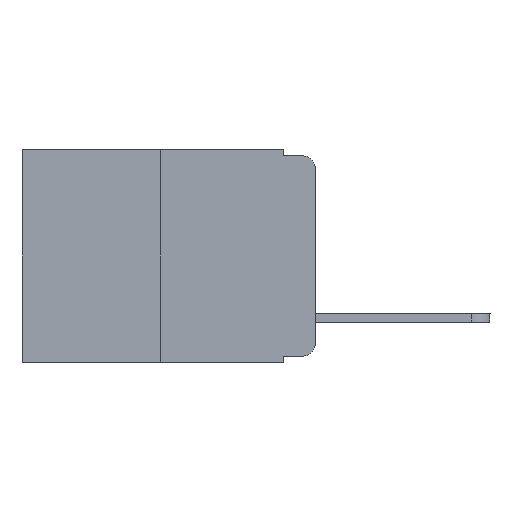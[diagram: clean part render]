
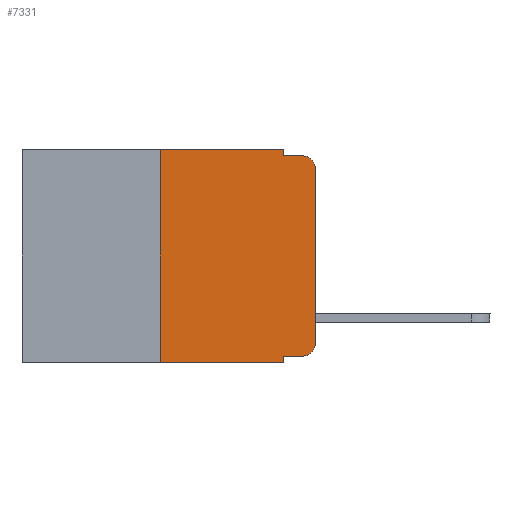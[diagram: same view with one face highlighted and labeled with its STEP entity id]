
A CAD part, left-side view. The second image highlights one B-rep face of the part: STEP entity #7331.
In plain terms, the highlighted planar face has unit normal (-1, 0, 0).
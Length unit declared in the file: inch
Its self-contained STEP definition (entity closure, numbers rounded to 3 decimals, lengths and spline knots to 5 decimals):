
#117 = CARTESIAN_POINT ( 'NONE',  ( 0., 0.473, 0. ) ) ;
#361 = VERTEX_POINT ( 'NONE', #13774 ) ;
#430 = DIRECTION ( 'NONE',  ( 1., 0., 0. ) ) ;
#773 = ORIENTED_EDGE ( 'NONE', *, *, #13720, .T. ) ;
#1698 = ORIENTED_EDGE ( 'NONE', *, *, #6007, .F. ) ;
#1771 = CARTESIAN_POINT ( 'NONE',  ( 0., 0.051, 0. ) ) ;
#1919 = CARTESIAN_POINT ( 'NONE',  ( 0., 0.051, -0.343 ) ) ;
#2036 = EDGE_CURVE ( 'NONE', #12910, #7004, #12169, .T. ) ;
#2043 = AXIS2_PLACEMENT_3D ( 'NONE', #8838, #430, #16953 ) ;
#2101 = VECTOR ( 'NONE', #10260, 39.37008 ) ;
#2117 = FACE_OUTER_BOUND ( 'NONE', #2971, .T. ) ;
#2604 = LINE ( 'NONE', #15202, #16610 ) ;
#2971 = EDGE_LOOP ( 'NONE', ( #773, #12628, #6554, #6378, #11436, #1698, #15024, #17090, #4696, #16770 ) ) ;
#3164 = EDGE_CURVE ( 'NONE', #16800, #361, #15571, .T. ) ;
#3185 = VERTEX_POINT ( 'NONE', #11881 ) ;
#3512 = CARTESIAN_POINT ( 'NONE',  ( 0., 0.02, -0.03 ) ) ;
#3571 = AXIS2_PLACEMENT_3D ( 'NONE', #11490, #14267, #6205 ) ;
#3693 = DIRECTION ( 'NONE',  ( -1., 0., 0. ) ) ;
#3844 = CARTESIAN_POINT ( 'NONE',  ( 0., 0.051, 0. ) ) ;
#3941 = VERTEX_POINT ( 'NONE', #5754 ) ;
#3953 = DIRECTION ( 'NONE',  ( 0., -1., 0. ) ) ;
#3967 = CARTESIAN_POINT ( 'NONE',  ( 0., 0.051, 0. ) ) ;
#4130 = VECTOR ( 'NONE', #16663, 39.37008 ) ;
#4312 = DIRECTION ( 'NONE',  ( 0., -1., 0. ) ) ;
#4548 = PLANE ( 'NONE',  #2043 ) ;
#4601 = DIRECTION ( 'NONE',  ( 0., 0., -1. ) ) ;
#4696 = ORIENTED_EDGE ( 'NONE', *, *, #11594, .T. ) ;
#4795 = VECTOR ( 'NONE', #3953, 39.37008 ) ;
#4859 = CARTESIAN_POINT ( 'NONE',  ( 0., 0., 0. ) ) ;
#4917 = LINE ( 'NONE', #117, #8762 ) ;
#5244 = VECTOR ( 'NONE', #4601, 39.37008 ) ;
#5399 = LINE ( 'NONE', #1771, #4130 ) ;
#5705 = LINE ( 'NONE', #10372, #2101 ) ;
#5754 = CARTESIAN_POINT ( 'NONE',  ( 0., 0.25, 0. ) ) ;
#6007 = EDGE_CURVE ( 'NONE', #8100, #3941, #2604, .T. ) ;
#6138 = VECTOR ( 'NONE', #13171, 39.37008 ) ;
#6205 = DIRECTION ( 'NONE',  ( 0., 0., -1. ) ) ;
#6206 = CARTESIAN_POINT ( 'NONE',  ( 0., 0.051, -0.333 ) ) ;
#6378 = ORIENTED_EDGE ( 'NONE', *, *, #9813, .F. ) ;
#6554 = ORIENTED_EDGE ( 'NONE', *, *, #8858, .F. ) ;
#7004 = VERTEX_POINT ( 'NONE', #10916 ) ;
#7331 = ADVANCED_FACE ( 'NONE', ( #2117 ), #4548, .F. ) ;
#7468 = EDGE_CURVE ( 'NONE', #8100, #15439, #5705, .T. ) ;
#7628 = VERTEX_POINT ( 'NONE', #3844 ) ;
#8100 = VERTEX_POINT ( 'NONE', #10708 ) ;
#8235 = LINE ( 'NONE', #3967, #5244 ) ;
#8433 = LINE ( 'NONE', #13370, #4795 ) ;
#8595 = AXIS2_PLACEMENT_3D ( 'NONE', #3512, #3693, #14429 ) ;
#8762 = VECTOR ( 'NONE', #10818, 39.37008 ) ;
#8838 = CARTESIAN_POINT ( 'NONE',  ( 0., 0.473, 0. ) ) ;
#8858 = EDGE_CURVE ( 'NONE', #3185, #361, #8433, .T. ) ;
#9759 = LINE ( 'NONE', #4859, #6138 ) ;
#9813 = EDGE_CURVE ( 'NONE', #7628, #3185, #5399, .T. ) ;
#10088 = VERTEX_POINT ( 'NONE', #6206 ) ;
#10260 = DIRECTION ( 'NONE',  ( 0., -1., 0. ) ) ;
#10372 = CARTESIAN_POINT ( 'NONE',  ( 0., 0.473, -0.343 ) ) ;
#10702 = EDGE_CURVE ( 'NONE', #3941, #7628, #4917, .T. ) ;
#10708 = CARTESIAN_POINT ( 'NONE',  ( 0., 0.25, -0.343 ) ) ;
#10818 = DIRECTION ( 'NONE',  ( 0., -1., 0. ) ) ;
#10827 = CARTESIAN_POINT ( 'NONE',  ( 0., 0., -0.03 ) ) ;
#10916 = CARTESIAN_POINT ( 'NONE',  ( 0., 0., -0.313 ) ) ;
#11158 = DIRECTION ( 'NONE',  ( 0., 0., 1. ) ) ;
#11436 = ORIENTED_EDGE ( 'NONE', *, *, #10702, .F. ) ;
#11490 = CARTESIAN_POINT ( 'NONE',  ( 0., 0.02, -0.313 ) ) ;
#11529 = VECTOR ( 'NONE', #4312, 39.37008 ) ;
#11594 = EDGE_CURVE ( 'NONE', #10088, #12910, #15138, .T. ) ;
#11881 = CARTESIAN_POINT ( 'NONE',  ( 0., 0.051, -0.01 ) ) ;
#12169 = CIRCLE ( 'NONE', #3571, 0.02 ) ;
#12628 = ORIENTED_EDGE ( 'NONE', *, *, #3164, .T. ) ;
#12910 = VERTEX_POINT ( 'NONE', #14028 ) ;
#13171 = DIRECTION ( 'NONE',  ( 0., 0., 1. ) ) ;
#13370 = CARTESIAN_POINT ( 'NONE',  ( 0., 0.051, -0.01 ) ) ;
#13720 = EDGE_CURVE ( 'NONE', #7004, #16800, #9759, .T. ) ;
#13774 = CARTESIAN_POINT ( 'NONE',  ( 0., 0.02, -0.01 ) ) ;
#14028 = CARTESIAN_POINT ( 'NONE',  ( 0., 0.02, -0.333 ) ) ;
#14267 = DIRECTION ( 'NONE',  ( -1., 0., 0. ) ) ;
#14429 = DIRECTION ( 'NONE',  ( 0., 0., -1. ) ) ;
#14648 = EDGE_CURVE ( 'NONE', #10088, #15439, #8235, .T. ) ;
#15024 = ORIENTED_EDGE ( 'NONE', *, *, #7468, .T. ) ;
#15138 = LINE ( 'NONE', #15414, #11529 ) ;
#15202 = CARTESIAN_POINT ( 'NONE',  ( 0., 0.25, 0. ) ) ;
#15414 = CARTESIAN_POINT ( 'NONE',  ( 0., 0.051, -0.333 ) ) ;
#15439 = VERTEX_POINT ( 'NONE', #1919 ) ;
#15571 = CIRCLE ( 'NONE', #8595, 0.02 ) ;
#16610 = VECTOR ( 'NONE', #11158, 39.37008 ) ;
#16663 = DIRECTION ( 'NONE',  ( 0., 0., -1. ) ) ;
#16770 = ORIENTED_EDGE ( 'NONE', *, *, #2036, .T. ) ;
#16800 = VERTEX_POINT ( 'NONE', #10827 ) ;
#16953 = DIRECTION ( 'NONE',  ( 0., 0., -1. ) ) ;
#17090 = ORIENTED_EDGE ( 'NONE', *, *, #14648, .F. ) ;
